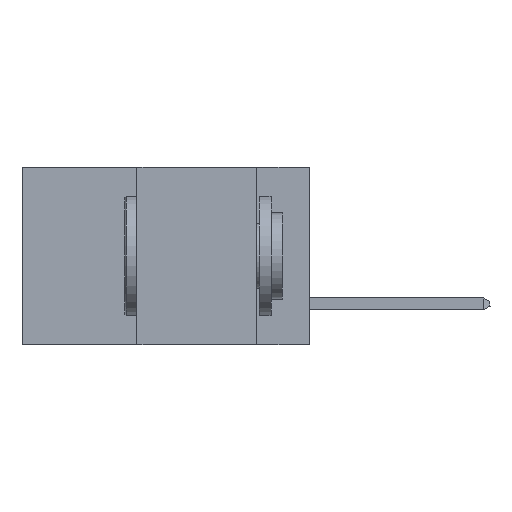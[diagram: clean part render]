
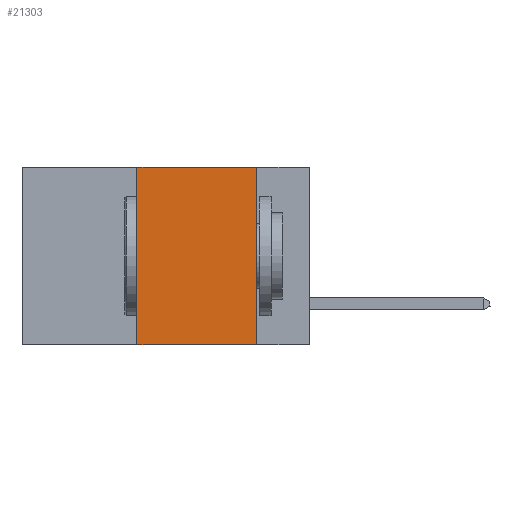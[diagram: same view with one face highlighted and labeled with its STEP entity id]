
A CAD part, left-side view. The second image highlights one B-rep face of the part: STEP entity #21303.
In plain terms, the highlighted planar face has unit normal (-1, 0, 0).
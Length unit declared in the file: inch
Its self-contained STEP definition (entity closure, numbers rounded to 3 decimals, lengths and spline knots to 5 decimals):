
#250 = CARTESIAN_POINT ( 'NONE',  ( 0., 0.11, -0.37 ) ) ;
#481 = LINE ( 'NONE', #23173, #9774 ) ;
#1955 = EDGE_CURVE ( 'NONE', #3371, #15793, #14010, .T. ) ;
#2093 = ORIENTED_EDGE ( 'NONE', *, *, #1955, .F. ) ;
#2304 = DIRECTION ( 'NONE',  ( 0., 0., 1. ) ) ;
#2929 = PLANE ( 'NONE',  #12151 ) ;
#3371 = VERTEX_POINT ( 'NONE', #9028 ) ;
#3417 = EDGE_LOOP ( 'NONE', ( #4101, #15665, #2093, #3821 ) ) ;
#3821 = ORIENTED_EDGE ( 'NONE', *, *, #11862, .T. ) ;
#4101 = ORIENTED_EDGE ( 'NONE', *, *, #22082, .F. ) ;
#6649 = DIRECTION ( 'NONE',  ( 0., 0., -1. ) ) ;
#6892 = VECTOR ( 'NONE', #9129, 39.37008 ) ;
#9028 = CARTESIAN_POINT ( 'NONE',  ( 0., 0.36, -0.37 ) ) ;
#9057 = CARTESIAN_POINT ( 'NONE',  ( 0., 0.6, -0.37 ) ) ;
#9096 = VECTOR ( 'NONE', #2304, 39.37008 ) ;
#9129 = DIRECTION ( 'NONE',  ( 0., -1., 0. ) ) ;
#9774 = VECTOR ( 'NONE', #21388, 39.37008 ) ;
#10866 = CARTESIAN_POINT ( 'NONE',  ( 0., 0.11, 0. ) ) ;
#11301 = VERTEX_POINT ( 'NONE', #250 ) ;
#11862 = EDGE_CURVE ( 'NONE', #3371, #11301, #12391, .T. ) ;
#12151 = AXIS2_PLACEMENT_3D ( 'NONE', #15835, #17662, #6649 ) ;
#12391 = LINE ( 'NONE', #9057, #6892 ) ;
#14010 = LINE ( 'NONE', #18276, #9096 ) ;
#14628 = EDGE_CURVE ( 'NONE', #15793, #16357, #481, .T. ) ;
#15665 = ORIENTED_EDGE ( 'NONE', *, *, #14628, .F. ) ;
#15793 = VERTEX_POINT ( 'NONE', #23631 ) ;
#15835 = CARTESIAN_POINT ( 'NONE',  ( 0., 0.6, 0. ) ) ;
#16357 = VERTEX_POINT ( 'NONE', #18113 ) ;
#17614 = LINE ( 'NONE', #10866, #22400 ) ;
#17662 = DIRECTION ( 'NONE',  ( 1., 0., 0. ) ) ;
#18113 = CARTESIAN_POINT ( 'NONE',  ( 0., 0.11, 0. ) ) ;
#18276 = CARTESIAN_POINT ( 'NONE',  ( 0., 0.36, 0. ) ) ;
#21303 = ADVANCED_FACE ( 'NONE', ( #21344 ), #2929, .F. ) ;
#21344 = FACE_OUTER_BOUND ( 'NONE', #3417, .T. ) ;
#21388 = DIRECTION ( 'NONE',  ( 0., -1., 0. ) ) ;
#21802 = DIRECTION ( 'NONE',  ( 0., 0., -1. ) ) ;
#22082 = EDGE_CURVE ( 'NONE', #16357, #11301, #17614, .T. ) ;
#22400 = VECTOR ( 'NONE', #21802, 39.37008 ) ;
#23173 = CARTESIAN_POINT ( 'NONE',  ( 0., 0.6, 0. ) ) ;
#23631 = CARTESIAN_POINT ( 'NONE',  ( 0., 0.36, 0. ) ) ;
